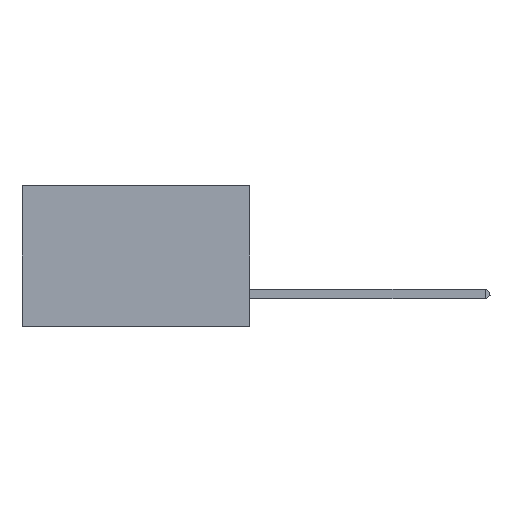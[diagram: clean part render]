
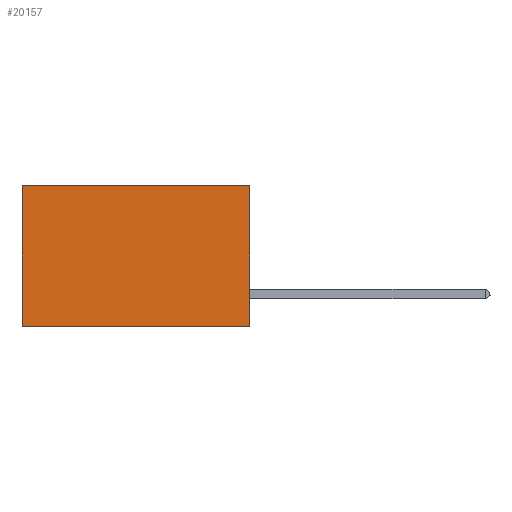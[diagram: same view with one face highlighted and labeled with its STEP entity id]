
A CAD part, left-side view. The second image highlights one B-rep face of the part: STEP entity #20157.
In plain terms, the highlighted planar face has unit normal (-1, 0, 0).
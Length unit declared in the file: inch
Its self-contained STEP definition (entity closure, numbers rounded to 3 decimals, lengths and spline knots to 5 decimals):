
#470 = VECTOR ( 'NONE', #22330, 39.37008 ) ;
#1981 = ORIENTED_EDGE ( 'NONE', *, *, #16916, .F. ) ;
#2002 = CARTESIAN_POINT ( 'NONE',  ( 0.2875, 0.6, -0.37 ) ) ;
#2621 = EDGE_CURVE ( 'NONE', #16067, #14642, #18717, .T. ) ;
#2950 = CARTESIAN_POINT ( 'NONE',  ( 0.2875, 0., 0. ) ) ;
#3530 = EDGE_LOOP ( 'NONE', ( #24715, #1981, #17969, #22276 ) ) ;
#4879 = LINE ( 'NONE', #9178, #9524 ) ;
#5705 = VECTOR ( 'NONE', #15319, 39.37008 ) ;
#6618 = AXIS2_PLACEMENT_3D ( 'NONE', #2950, #20749, #17206 ) ;
#6881 = VECTOR ( 'NONE', #14032, 39.37008 ) ;
#6978 = CARTESIAN_POINT ( 'NONE',  ( 0.2875, 0., -0.37 ) ) ;
#8331 = CARTESIAN_POINT ( 'NONE',  ( 0.2875, 0.6, 0. ) ) ;
#8444 = CARTESIAN_POINT ( 'NONE',  ( 0.2875, 0., 0. ) ) ;
#9178 = CARTESIAN_POINT ( 'NONE',  ( 0.2875, 0.6, 0. ) ) ;
#9524 = VECTOR ( 'NONE', #15183, 39.37008 ) ;
#11000 = LINE ( 'NONE', #19252, #5705 ) ;
#11400 = CARTESIAN_POINT ( 'NONE',  ( 0.2875, 0., 0. ) ) ;
#11731 = EDGE_CURVE ( 'NONE', #14642, #14525, #4879, .T. ) ;
#11809 = FACE_OUTER_BOUND ( 'NONE', #3530, .T. ) ;
#12638 = LINE ( 'NONE', #8444, #470 ) ;
#14032 = DIRECTION ( 'NONE',  ( 0., 1., 0. ) ) ;
#14525 = VERTEX_POINT ( 'NONE', #2002 ) ;
#14642 = VERTEX_POINT ( 'NONE', #8331 ) ;
#15183 = DIRECTION ( 'NONE',  ( 0., 0., -1. ) ) ;
#15319 = DIRECTION ( 'NONE',  ( 0., 1., 0. ) ) ;
#16067 = VERTEX_POINT ( 'NONE', #11400 ) ;
#16869 = VERTEX_POINT ( 'NONE', #6978 ) ;
#16916 = EDGE_CURVE ( 'NONE', #16869, #14525, #11000, .T. ) ;
#17206 = DIRECTION ( 'NONE',  ( 0., 0., -1. ) ) ;
#17969 = ORIENTED_EDGE ( 'NONE', *, *, #22436, .F. ) ;
#18717 = LINE ( 'NONE', #19471, #6881 ) ;
#18725 = PLANE ( 'NONE',  #6618 ) ;
#19252 = CARTESIAN_POINT ( 'NONE',  ( 0.2875, 0., -0.37 ) ) ;
#19471 = CARTESIAN_POINT ( 'NONE',  ( 0.2875, 0., 0. ) ) ;
#20157 = ADVANCED_FACE ( 'NONE', ( #11809 ), #18725, .F. ) ;
#20749 = DIRECTION ( 'NONE',  ( 1., 0., 0. ) ) ;
#22276 = ORIENTED_EDGE ( 'NONE', *, *, #2621, .T. ) ;
#22330 = DIRECTION ( 'NONE',  ( 0., 0., -1. ) ) ;
#22436 = EDGE_CURVE ( 'NONE', #16067, #16869, #12638, .T. ) ;
#24715 = ORIENTED_EDGE ( 'NONE', *, *, #11731, .T. ) ;
